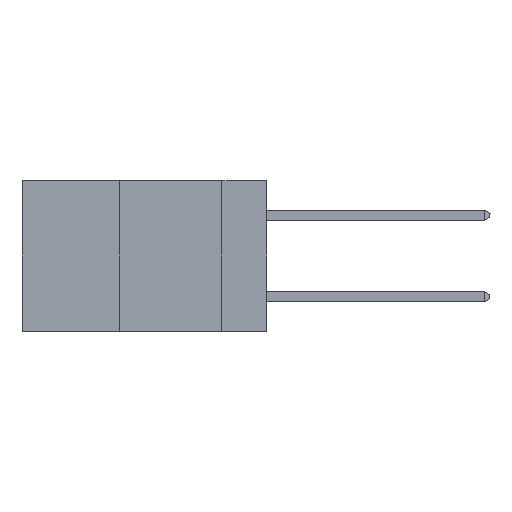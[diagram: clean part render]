
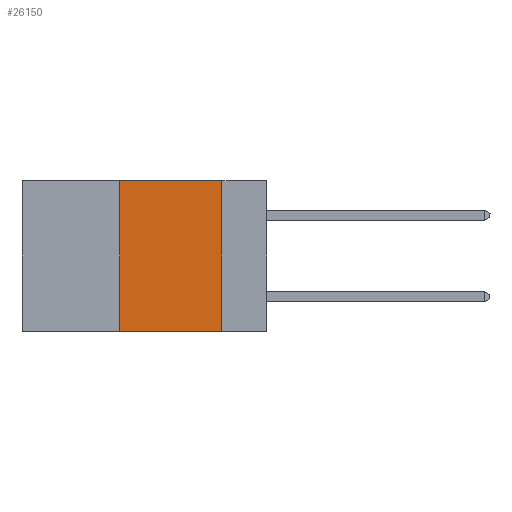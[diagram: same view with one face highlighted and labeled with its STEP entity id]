
A CAD part, left-side view. The second image highlights one B-rep face of the part: STEP entity #26150.
In plain terms, the highlighted planar face has unit normal (-1, 0, 0).
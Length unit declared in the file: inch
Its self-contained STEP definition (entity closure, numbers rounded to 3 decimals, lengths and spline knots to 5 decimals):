
#1299 = CARTESIAN_POINT ( 'NONE',  ( 0., 0.11, 0. ) ) ;
#4541 = AXIS2_PLACEMENT_3D ( 'NONE', #7425, #22930, #5658 ) ;
#5658 = DIRECTION ( 'NONE',  ( 0., 0., -1. ) ) ;
#5666 = VECTOR ( 'NONE', #29558, 39.37008 ) ;
#7425 = CARTESIAN_POINT ( 'NONE',  ( 0., 0.6, 0. ) ) ;
#7679 = LINE ( 'NONE', #33127, #36837 ) ;
#9301 = CARTESIAN_POINT ( 'NONE',  ( 0., 0.11, 0. ) ) ;
#9480 = CARTESIAN_POINT ( 'NONE',  ( 0., 0.6, 0. ) ) ;
#9662 = EDGE_CURVE ( 'NONE', #11161, #14833, #37079, .T. ) ;
#11161 = VERTEX_POINT ( 'NONE', #30227 ) ;
#11539 = DIRECTION ( 'NONE',  ( 0., 0., -1. ) ) ;
#14833 = VERTEX_POINT ( 'NONE', #9301 ) ;
#15183 = ORIENTED_EDGE ( 'NONE', *, *, #33345, .T. ) ;
#16591 = CARTESIAN_POINT ( 'NONE',  ( 0., 0.11, -0.37 ) ) ;
#18313 = CARTESIAN_POINT ( 'NONE',  ( 0., 0.6, -0.37 ) ) ;
#19257 = PLANE ( 'NONE',  #4541 ) ;
#19411 = ORIENTED_EDGE ( 'NONE', *, *, #20408, .F. ) ;
#19652 = ORIENTED_EDGE ( 'NONE', *, *, #19993, .F. ) ;
#19960 = VECTOR ( 'NONE', #20338, 39.37008 ) ;
#19993 = EDGE_CURVE ( 'NONE', #20589, #11161, #7679, .T. ) ;
#20338 = DIRECTION ( 'NONE',  ( 0., -1., 0. ) ) ;
#20408 = EDGE_CURVE ( 'NONE', #14833, #29430, #21759, .T. ) ;
#20589 = VERTEX_POINT ( 'NONE', #35640 ) ;
#21759 = LINE ( 'NONE', #1299, #22671 ) ;
#21760 = LINE ( 'NONE', #18313, #19960 ) ;
#22671 = VECTOR ( 'NONE', #11539, 39.37008 ) ;
#22930 = DIRECTION ( 'NONE',  ( 1., 0., 0. ) ) ;
#24415 = EDGE_LOOP ( 'NONE', ( #19411, #26835, #19652, #15183 ) ) ;
#26150 = ADVANCED_FACE ( 'NONE', ( #36018 ), #19257, .F. ) ;
#26835 = ORIENTED_EDGE ( 'NONE', *, *, #9662, .F. ) ;
#29430 = VERTEX_POINT ( 'NONE', #16591 ) ;
#29558 = DIRECTION ( 'NONE',  ( 0., -1., 0. ) ) ;
#30227 = CARTESIAN_POINT ( 'NONE',  ( 0., 0.36, 0. ) ) ;
#33127 = CARTESIAN_POINT ( 'NONE',  ( 0., 0.36, 0. ) ) ;
#33345 = EDGE_CURVE ( 'NONE', #20589, #29430, #21760, .T. ) ;
#35640 = CARTESIAN_POINT ( 'NONE',  ( 0., 0.36, -0.37 ) ) ;
#36018 = FACE_OUTER_BOUND ( 'NONE', #24415, .T. ) ;
#36730 = DIRECTION ( 'NONE',  ( 0., 0., 1. ) ) ;
#36837 = VECTOR ( 'NONE', #36730, 39.37008 ) ;
#37079 = LINE ( 'NONE', #9480, #5666 ) ;
